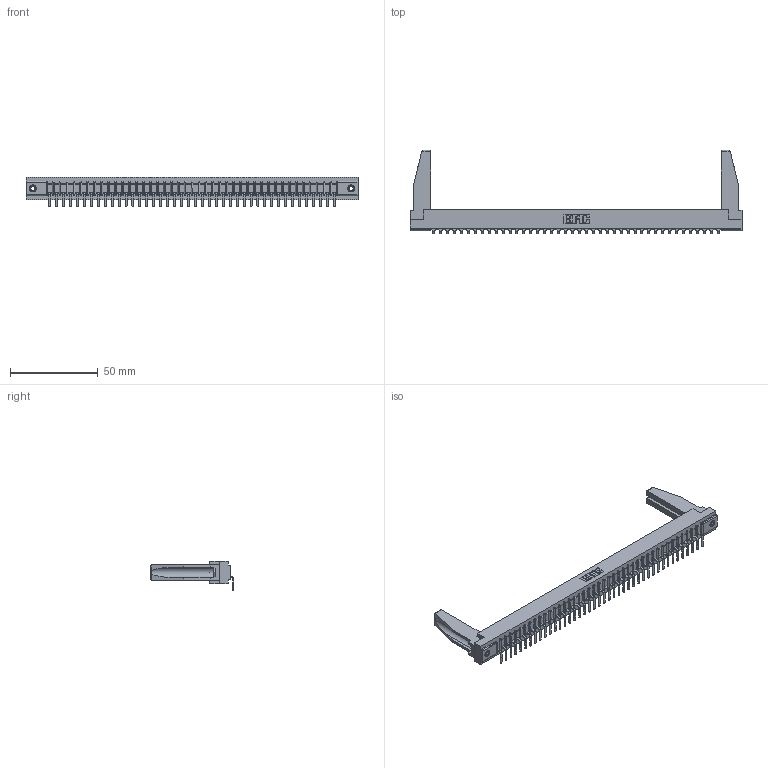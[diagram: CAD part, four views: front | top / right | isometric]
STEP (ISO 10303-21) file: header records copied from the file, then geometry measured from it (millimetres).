
FILE_DESCRIPTION (( 'STEP AP203' ), '1' );
FILE_NAME ('357-042-559-178.STEP', '2022-07-12T19:37:39', ( '' ), ( '' ), 'SwSTEP 2.0', 'SolidWorks 2020', '' );
FILE_SCHEMA (( 'CONFIG_CONTROL_DESIGN' ));
Length unit declared in the file: inch
Products named in the file (5): 307-290-001_558 559 - 1 (Single); 345-250-001_345-250-001-102; 307 Part_.156 Dia Mounting Holes; 307-220-078; 357-042-559-178
Assembly tree (47 placements, depth 2):
  357-042-559-178
    307 Part_.156 Dia Mounting Holes
    307-290-001_558 559 - 1 (Single)  x42
    307-220-078  x2
    345-250-001_345-250-001-102  x2
Bounding box: 189.43 x 47.41 x 16.8 mm (x, y, z)
Volume: 23681.8 mm3; surface area: 24789.1 mm2
Topology: 47 solids, 47 shells, 2811 faces, 7961 edges, 5126 vertices
Faces by surface type: plane 1792, cylinder 917, sphere 86, cone 12, torus 4
Entity records: 38549 total; most frequent: CARTESIAN_POINT 6494, ORIENTED_EDGE 6436, DIRECTION 6272, EDGE_CURVE 3218, VECTOR 2472, LINE 2472, VERTEX_POINT 2080, AXIS2_PLACEMENT_3D 1900
